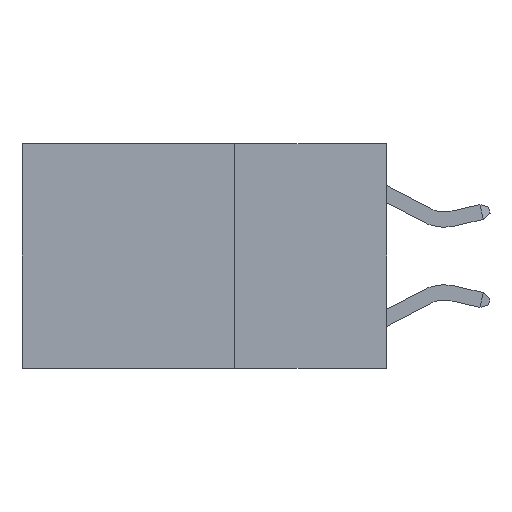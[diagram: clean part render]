
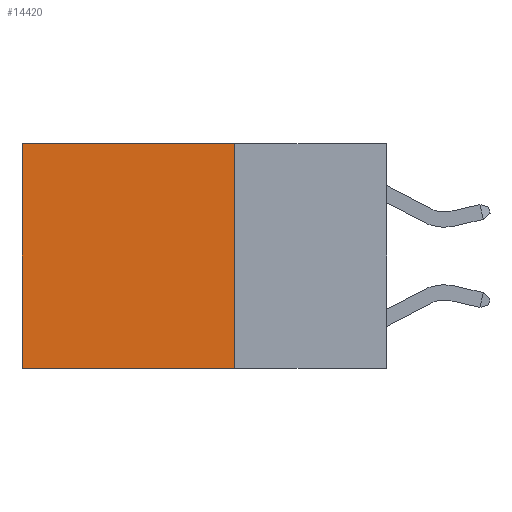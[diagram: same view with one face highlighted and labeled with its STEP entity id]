
A CAD part, left-side view. The second image highlights one B-rep face of the part: STEP entity #14420.
In plain terms, the highlighted planar face has unit normal (-1, 0, 0).
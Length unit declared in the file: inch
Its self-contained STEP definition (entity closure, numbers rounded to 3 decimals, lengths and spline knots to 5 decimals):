
#1117 = VERTEX_POINT ( 'NONE', #17791 ) ;
#1652 = VECTOR ( 'NONE', #20400, 39.37008 ) ;
#1735 = VERTEX_POINT ( 'NONE', #2650 ) ;
#2590 = VECTOR ( 'NONE', #13978, 39.37008 ) ;
#2650 = CARTESIAN_POINT ( 'NONE',  ( 0.2625, 0.25, -0.37 ) ) ;
#3010 = ORIENTED_EDGE ( 'NONE', *, *, #19920, .T. ) ;
#4469 = PLANE ( 'NONE',  #12455 ) ;
#4542 = CARTESIAN_POINT ( 'NONE',  ( 0.2625, 0.25, -0.37 ) ) ;
#5814 = ORIENTED_EDGE ( 'NONE', *, *, #18820, .F. ) ;
#7185 = CARTESIAN_POINT ( 'NONE',  ( 0.2625, 0.6, 0. ) ) ;
#7356 = LINE ( 'NONE', #8750, #2590 ) ;
#7650 = ORIENTED_EDGE ( 'NONE', *, *, #16954, .T. ) ;
#8058 = DIRECTION ( 'NONE',  ( 0., 0., -1. ) ) ;
#8628 = EDGE_CURVE ( 'NONE', #1117, #1735, #16735, .T. ) ;
#8750 = CARTESIAN_POINT ( 'NONE',  ( 0.2625, 0.25, 0. ) ) ;
#9751 = CARTESIAN_POINT ( 'NONE',  ( 0.2625, 0.6, -0.37 ) ) ;
#10352 = DIRECTION ( 'NONE',  ( 0., 0., -1. ) ) ;
#10468 = ORIENTED_EDGE ( 'NONE', *, *, #8628, .F. ) ;
#12455 = AXIS2_PLACEMENT_3D ( 'NONE', #13227, #16836, #8058 ) ;
#13227 = CARTESIAN_POINT ( 'NONE',  ( 0.2625, 0.25, 0. ) ) ;
#13787 = CARTESIAN_POINT ( 'NONE',  ( 0.2625, 0.6, 0. ) ) ;
#13978 = DIRECTION ( 'NONE',  ( 0., 1., 0. ) ) ;
#14420 = ADVANCED_FACE ( 'NONE', ( #22424 ), #4469, .F. ) ;
#14676 = VECTOR ( 'NONE', #18620, 39.37008 ) ;
#15049 = VECTOR ( 'NONE', #10352, 39.37008 ) ;
#16735 = LINE ( 'NONE', #19184, #15049 ) ;
#16836 = DIRECTION ( 'NONE',  ( 1., 0., 0. ) ) ;
#16954 = EDGE_CURVE ( 'NONE', #1117, #18128, #7356, .T. ) ;
#17791 = CARTESIAN_POINT ( 'NONE',  ( 0.2625, 0.25, 0. ) ) ;
#18128 = VERTEX_POINT ( 'NONE', #7185 ) ;
#18620 = DIRECTION ( 'NONE',  ( 0., 0., -1. ) ) ;
#18820 = EDGE_CURVE ( 'NONE', #1735, #22089, #21066, .T. ) ;
#19184 = CARTESIAN_POINT ( 'NONE',  ( 0.2625, 0.25, 0. ) ) ;
#19397 = LINE ( 'NONE', #13787, #14676 ) ;
#19920 = EDGE_CURVE ( 'NONE', #18128, #22089, #19397, .T. ) ;
#20400 = DIRECTION ( 'NONE',  ( 0., 1., 0. ) ) ;
#21066 = LINE ( 'NONE', #4542, #1652 ) ;
#21600 = EDGE_LOOP ( 'NONE', ( #3010, #5814, #10468, #7650 ) ) ;
#22089 = VERTEX_POINT ( 'NONE', #9751 ) ;
#22424 = FACE_OUTER_BOUND ( 'NONE', #21600, .T. ) ;
